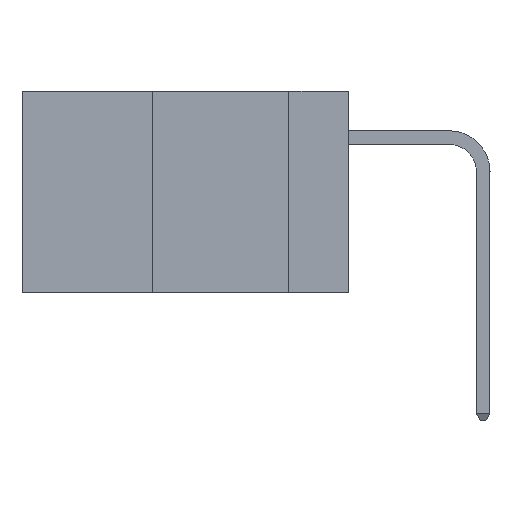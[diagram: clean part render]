
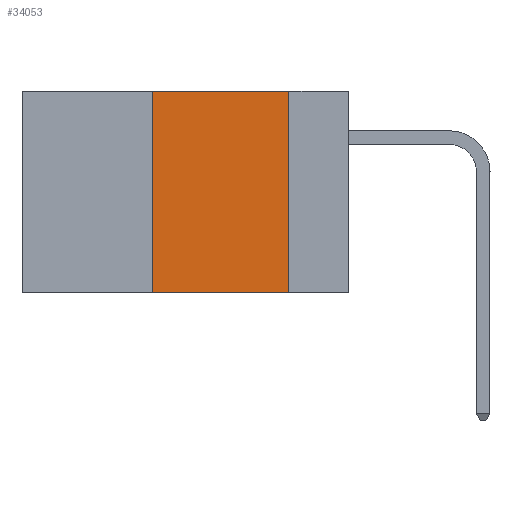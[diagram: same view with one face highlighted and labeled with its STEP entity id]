
A CAD part, left-side view. The second image highlights one B-rep face of the part: STEP entity #34053.
In plain terms, the highlighted planar face has unit normal (-1, 0, 0).
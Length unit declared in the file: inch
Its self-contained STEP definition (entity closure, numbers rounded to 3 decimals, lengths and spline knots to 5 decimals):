
#1534 = VECTOR ( 'NONE', #9615, 39.37008 ) ;
#4025 = CARTESIAN_POINT ( 'NONE',  ( 0., 0.36, 0. ) ) ;
#6333 = LINE ( 'NONE', #4025, #35585 ) ;
#7645 = DIRECTION ( 'NONE',  ( 0., 0., 1. ) ) ;
#8889 = LINE ( 'NONE', #31121, #1534 ) ;
#9063 = DIRECTION ( 'NONE',  ( 0., -1., 0. ) ) ;
#9615 = DIRECTION ( 'NONE',  ( 0., -1., 0. ) ) ;
#10927 = ORIENTED_EDGE ( 'NONE', *, *, #46587, .T. ) ;
#11758 = ORIENTED_EDGE ( 'NONE', *, *, #32774, .F. ) ;
#12099 = ORIENTED_EDGE ( 'NONE', *, *, #24988, .F. ) ;
#13049 = VERTEX_POINT ( 'NONE', #32064 ) ;
#14006 = DIRECTION ( 'NONE',  ( 0., 0., -1. ) ) ;
#14857 = PLANE ( 'NONE',  #21303 ) ;
#21215 = VERTEX_POINT ( 'NONE', #36093 ) ;
#21303 = AXIS2_PLACEMENT_3D ( 'NONE', #29453, #25707, #44396 ) ;
#24812 = VECTOR ( 'NONE', #9063, 39.37008 ) ;
#24988 = EDGE_CURVE ( 'NONE', #35270, #13049, #34371, .T. ) ;
#25707 = DIRECTION ( 'NONE',  ( 1., 0., 0. ) ) ;
#29140 = FACE_OUTER_BOUND ( 'NONE', #43208, .T. ) ;
#29147 = ORIENTED_EDGE ( 'NONE', *, *, #29306, .F. ) ;
#29306 = EDGE_CURVE ( 'NONE', #21215, #35270, #6333, .T. ) ;
#29453 = CARTESIAN_POINT ( 'NONE',  ( 0., 0.6, 0. ) ) ;
#30254 = LINE ( 'NONE', #35221, #42121 ) ;
#31121 = CARTESIAN_POINT ( 'NONE',  ( 0., 0.6, -0.37 ) ) ;
#32064 = CARTESIAN_POINT ( 'NONE',  ( 0., 0.11, 0. ) ) ;
#32774 = EDGE_CURVE ( 'NONE', #13049, #40354, #30254, .T. ) ;
#34053 = ADVANCED_FACE ( 'NONE', ( #29140 ), #14857, .F. ) ;
#34371 = LINE ( 'NONE', #41304, #24812 ) ;
#35221 = CARTESIAN_POINT ( 'NONE',  ( 0., 0.11, 0. ) ) ;
#35270 = VERTEX_POINT ( 'NONE', #38047 ) ;
#35585 = VECTOR ( 'NONE', #7645, 39.37008 ) ;
#36093 = CARTESIAN_POINT ( 'NONE',  ( 0., 0.36, -0.37 ) ) ;
#38047 = CARTESIAN_POINT ( 'NONE',  ( 0., 0.36, 0. ) ) ;
#40354 = VERTEX_POINT ( 'NONE', #46141 ) ;
#41304 = CARTESIAN_POINT ( 'NONE',  ( 0., 0.6, 0. ) ) ;
#42121 = VECTOR ( 'NONE', #14006, 39.37008 ) ;
#43208 = EDGE_LOOP ( 'NONE', ( #11758, #12099, #29147, #10927 ) ) ;
#44396 = DIRECTION ( 'NONE',  ( 0., 0., -1. ) ) ;
#46141 = CARTESIAN_POINT ( 'NONE',  ( 0., 0.11, -0.37 ) ) ;
#46587 = EDGE_CURVE ( 'NONE', #21215, #40354, #8889, .T. ) ;
